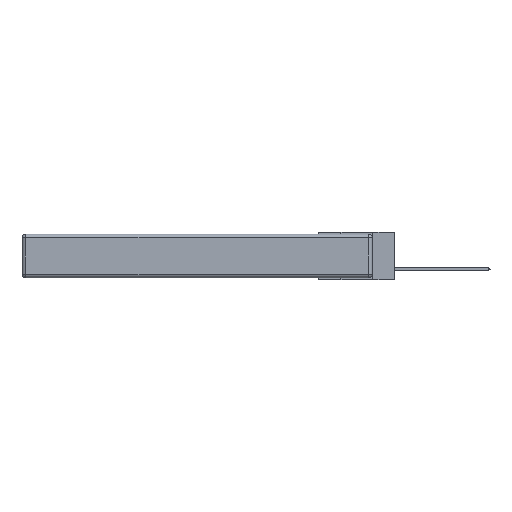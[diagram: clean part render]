
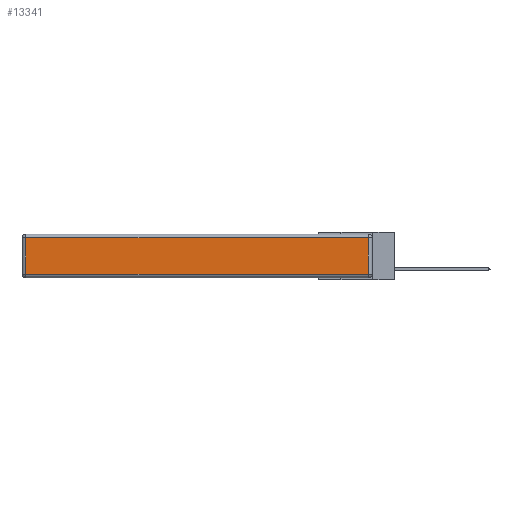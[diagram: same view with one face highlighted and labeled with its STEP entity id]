
A CAD part, left-side view. The second image highlights one B-rep face of the part: STEP entity #13341.
In plain terms, the highlighted planar face has unit normal (-1, 0, 0).
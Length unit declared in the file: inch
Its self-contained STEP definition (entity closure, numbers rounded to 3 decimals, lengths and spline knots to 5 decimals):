
#326 = DIRECTION ( 'NONE',  ( -1., 0., 0. ) ) ;
#383 = AXIS2_PLACEMENT_3D ( 'NONE', #3618, #326, #1327 ) ;
#1327 = DIRECTION ( 'NONE',  ( 0., 0., 1. ) ) ;
#1429 = CARTESIAN_POINT ( 'NONE',  ( 0., 0.03, -0.03 ) ) ;
#1538 = EDGE_LOOP ( 'NONE', ( #4583, #5156, #12527, #9492 ) ) ;
#1688 = DIRECTION ( 'NONE',  ( 0., 0., -1. ) ) ;
#1749 = VERTEX_POINT ( 'NONE', #5554 ) ;
#2511 = PLANE ( 'NONE',  #383 ) ;
#2525 = DIRECTION ( 'NONE',  ( 0., 1., 0. ) ) ;
#2764 = FACE_OUTER_BOUND ( 'NONE', #1538, .T. ) ;
#2772 = DIRECTION ( 'NONE',  ( 0., -1., 0. ) ) ;
#3165 = VECTOR ( 'NONE', #1688, 39.37008 ) ;
#3543 = VECTOR ( 'NONE', #13026, 39.37008 ) ;
#3618 = CARTESIAN_POINT ( 'NONE',  ( 0., 0., -0.343 ) ) ;
#3846 = LINE ( 'NONE', #9376, #7400 ) ;
#3874 = CARTESIAN_POINT ( 'NONE',  ( 0., 2.72, -0.343 ) ) ;
#4583 = ORIENTED_EDGE ( 'NONE', *, *, #11424, .T. ) ;
#5156 = ORIENTED_EDGE ( 'NONE', *, *, #11782, .T. ) ;
#5498 = LINE ( 'NONE', #8451, #8000 ) ;
#5529 = VERTEX_POINT ( 'NONE', #1429 ) ;
#5554 = CARTESIAN_POINT ( 'NONE',  ( 0., 0.03, -0.313 ) ) ;
#6466 = VERTEX_POINT ( 'NONE', #6845 ) ;
#6845 = CARTESIAN_POINT ( 'NONE',  ( 0., 2.72, -0.03 ) ) ;
#7245 = VERTEX_POINT ( 'NONE', #7746 ) ;
#7400 = VECTOR ( 'NONE', #2525, 39.37008 ) ;
#7746 = CARTESIAN_POINT ( 'NONE',  ( 0., 2.72, -0.313 ) ) ;
#8000 = VECTOR ( 'NONE', #2772, 39.37008 ) ;
#8451 = CARTESIAN_POINT ( 'NONE',  ( 0., 0., -0.313 ) ) ;
#8875 = LINE ( 'NONE', #3874, #3165 ) ;
#9376 = CARTESIAN_POINT ( 'NONE',  ( 0., 2.75, -0.03 ) ) ;
#9492 = ORIENTED_EDGE ( 'NONE', *, *, #12016, .T. ) ;
#11424 = EDGE_CURVE ( 'NONE', #7245, #1749, #5498, .T. ) ;
#11782 = EDGE_CURVE ( 'NONE', #1749, #5529, #12900, .T. ) ;
#12016 = EDGE_CURVE ( 'NONE', #6466, #7245, #8875, .T. ) ;
#12527 = ORIENTED_EDGE ( 'NONE', *, *, #13199, .T. ) ;
#12900 = LINE ( 'NONE', #14158, #3543 ) ;
#13026 = DIRECTION ( 'NONE',  ( 0., 0., 1. ) ) ;
#13199 = EDGE_CURVE ( 'NONE', #5529, #6466, #3846, .T. ) ;
#13341 = ADVANCED_FACE ( 'NONE', ( #2764 ), #2511, .T. ) ;
#14158 = CARTESIAN_POINT ( 'NONE',  ( 0., 0.03, -0.343 ) ) ;
